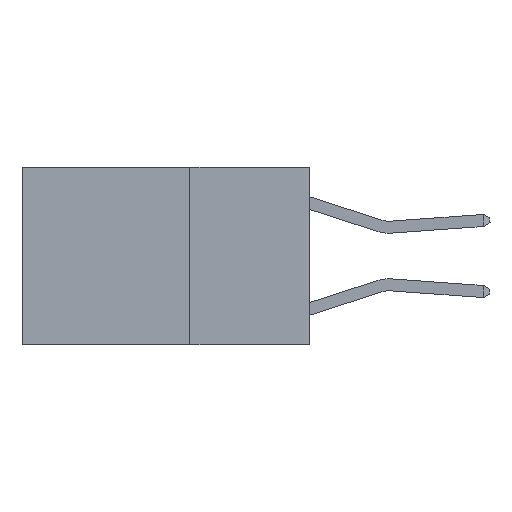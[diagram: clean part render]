
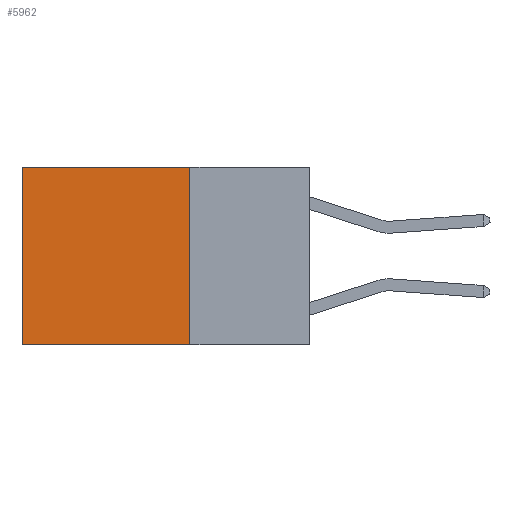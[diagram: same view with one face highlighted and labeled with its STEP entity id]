
A CAD part, left-side view. The second image highlights one B-rep face of the part: STEP entity #5962.
In plain terms, the highlighted planar face has unit normal (-1, 0, 0).
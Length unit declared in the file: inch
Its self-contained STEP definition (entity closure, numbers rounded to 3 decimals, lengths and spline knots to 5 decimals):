
#156 = EDGE_CURVE ( 'NONE', #7300, #5420, #6554, .T. ) ;
#673 = DIRECTION ( 'NONE',  ( 0., 0., -1. ) ) ;
#1779 = CARTESIAN_POINT ( 'NONE',  ( 0.2625, 0.25, 0. ) ) ;
#2039 = ORIENTED_EDGE ( 'NONE', *, *, #4455, .T. ) ;
#2175 = EDGE_CURVE ( 'NONE', #8283, #4829, #12779, .T. ) ;
#2760 = CARTESIAN_POINT ( 'NONE',  ( 0.2625, 0.6, -0.37 ) ) ;
#3202 = EDGE_CURVE ( 'NONE', #8283, #7300, #13293, .T. ) ;
#4168 = VECTOR ( 'NONE', #13096, 39.37008 ) ;
#4405 = EDGE_LOOP ( 'NONE', ( #2039, #9273, #10341, #5976 ) ) ;
#4455 = EDGE_CURVE ( 'NONE', #4829, #5420, #5648, .T. ) ;
#4733 = PLANE ( 'NONE',  #11599 ) ;
#4829 = VERTEX_POINT ( 'NONE', #13170 ) ;
#5420 = VERTEX_POINT ( 'NONE', #2760 ) ;
#5648 = LINE ( 'NONE', #5986, #11067 ) ;
#5802 = DIRECTION ( 'NONE',  ( 1., 0., 0. ) ) ;
#5962 = ADVANCED_FACE ( 'NONE', ( #8821 ), #4733, .F. ) ;
#5976 = ORIENTED_EDGE ( 'NONE', *, *, #2175, .T. ) ;
#5986 = CARTESIAN_POINT ( 'NONE',  ( 0.2625, 0.6, 0. ) ) ;
#6554 = LINE ( 'NONE', #10954, #11995 ) ;
#7215 = CARTESIAN_POINT ( 'NONE',  ( 0.2625, 0.25, 0. ) ) ;
#7300 = VERTEX_POINT ( 'NONE', #12490 ) ;
#7704 = DIRECTION ( 'NONE',  ( 0., 1., 0. ) ) ;
#8283 = VERTEX_POINT ( 'NONE', #7215 ) ;
#8821 = FACE_OUTER_BOUND ( 'NONE', #4405, .T. ) ;
#9247 = DIRECTION ( 'NONE',  ( 0., 0., -1. ) ) ;
#9273 = ORIENTED_EDGE ( 'NONE', *, *, #156, .F. ) ;
#9733 = VECTOR ( 'NONE', #673, 39.37008 ) ;
#10341 = ORIENTED_EDGE ( 'NONE', *, *, #3202, .F. ) ;
#10954 = CARTESIAN_POINT ( 'NONE',  ( 0.2625, 0.25, -0.37 ) ) ;
#11067 = VECTOR ( 'NONE', #9247, 39.37008 ) ;
#11599 = AXIS2_PLACEMENT_3D ( 'NONE', #12287, #5802, #13368 ) ;
#11995 = VECTOR ( 'NONE', #7704, 39.37008 ) ;
#12022 = CARTESIAN_POINT ( 'NONE',  ( 0.2625, 0.25, 0. ) ) ;
#12287 = CARTESIAN_POINT ( 'NONE',  ( 0.2625, 0.25, 0. ) ) ;
#12490 = CARTESIAN_POINT ( 'NONE',  ( 0.2625, 0.25, -0.37 ) ) ;
#12779 = LINE ( 'NONE', #12022, #4168 ) ;
#13096 = DIRECTION ( 'NONE',  ( 0., 1., 0. ) ) ;
#13170 = CARTESIAN_POINT ( 'NONE',  ( 0.2625, 0.6, 0. ) ) ;
#13293 = LINE ( 'NONE', #1779, #9733 ) ;
#13368 = DIRECTION ( 'NONE',  ( 0., 0., -1. ) ) ;
